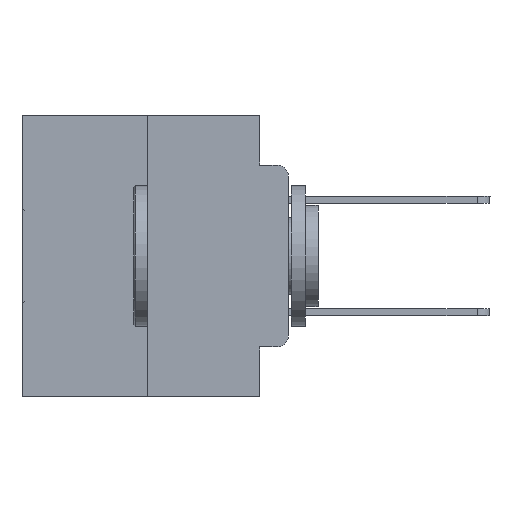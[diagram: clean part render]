
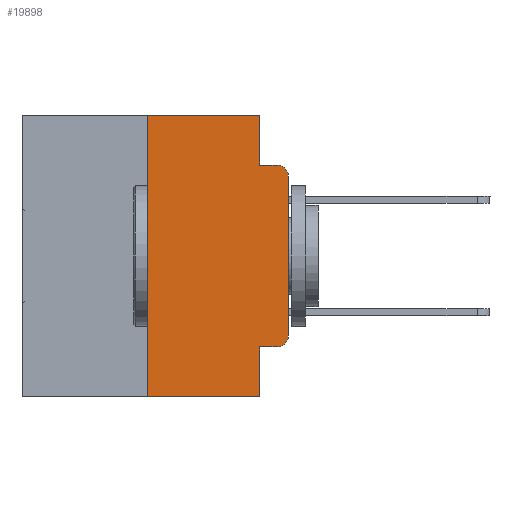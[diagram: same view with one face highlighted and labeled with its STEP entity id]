
A CAD part, left-side view. The second image highlights one B-rep face of the part: STEP entity #19898.
In plain terms, the highlighted planar face has unit normal (-1, 0, 0).
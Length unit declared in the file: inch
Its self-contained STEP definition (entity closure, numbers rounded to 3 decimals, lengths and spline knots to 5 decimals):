
#497 = EDGE_CURVE ( 'NONE', #6407, #11371, #31615, .T. ) ;
#2572 = CARTESIAN_POINT ( 'NONE',  ( 0., 0.02, -0.1085 ) ) ;
#3249 = CARTESIAN_POINT ( 'NONE',  ( 0., 0.473, 0. ) ) ;
#3807 = AXIS2_PLACEMENT_3D ( 'NONE', #2572, #20241, #5185 ) ;
#3982 = CARTESIAN_POINT ( 'NONE',  ( 0., 0.051, 0. ) ) ;
#4073 = CARTESIAN_POINT ( 'NONE',  ( 0., 0.02, -0.0885 ) ) ;
#4460 = VECTOR ( 'NONE', #25792, 39.37008 ) ;
#5185 = DIRECTION ( 'NONE',  ( 0., 0., -1. ) ) ;
#5262 = LINE ( 'NONE', #18296, #4460 ) ;
#5827 = DIRECTION ( 'NONE',  ( 0., 0., -1. ) ) ;
#6192 = VECTOR ( 'NONE', #22529, 39.37008 ) ;
#6322 = VERTEX_POINT ( 'NONE', #23904 ) ;
#6380 = VECTOR ( 'NONE', #16182, 39.37008 ) ;
#6407 = VERTEX_POINT ( 'NONE', #23125 ) ;
#6460 = CARTESIAN_POINT ( 'NONE',  ( 0., 0.25, 0. ) ) ;
#7505 = EDGE_CURVE ( 'NONE', #6407, #19344, #25253, .T. ) ;
#7971 = LINE ( 'NONE', #28502, #6380 ) ;
#8475 = ORIENTED_EDGE ( 'NONE', *, *, #19273, .T. ) ;
#8670 = CARTESIAN_POINT ( 'NONE',  ( 0., 0.051, -0.5 ) ) ;
#8671 = CARTESIAN_POINT ( 'NONE',  ( 0., 0.051, 0. ) ) ;
#8847 = EDGE_CURVE ( 'NONE', #10869, #28067, #17464, .T. ) ;
#9014 = AXIS2_PLACEMENT_3D ( 'NONE', #3249, #20863, #5827 ) ;
#9240 = EDGE_CURVE ( 'NONE', #13804, #10869, #7971, .T. ) ;
#9842 = CARTESIAN_POINT ( 'NONE',  ( 0., 0.473, 0. ) ) ;
#9876 = ORIENTED_EDGE ( 'NONE', *, *, #7505, .F. ) ;
#10343 = DIRECTION ( 'NONE',  ( -1., 0., 0. ) ) ;
#10869 = VERTEX_POINT ( 'NONE', #6460 ) ;
#11147 = CARTESIAN_POINT ( 'NONE',  ( 0., 0.02, -0.4115 ) ) ;
#11371 = VERTEX_POINT ( 'NONE', #11147 ) ;
#11706 = LINE ( 'NONE', #15580, #16750 ) ;
#11901 = VECTOR ( 'NONE', #30129, 39.37008 ) ;
#12413 = DIRECTION ( 'NONE',  ( 0., -1., 0. ) ) ;
#12712 = ORIENTED_EDGE ( 'NONE', *, *, #497, .T. ) ;
#13409 = PLANE ( 'NONE',  #9014 ) ;
#13804 = VERTEX_POINT ( 'NONE', #18641 ) ;
#14194 = VERTEX_POINT ( 'NONE', #17664 ) ;
#14289 = EDGE_CURVE ( 'NONE', #28067, #14194, #11706, .T. ) ;
#15580 = CARTESIAN_POINT ( 'NONE',  ( 0., 0.051, 0. ) ) ;
#15982 = EDGE_CURVE ( 'NONE', #14194, #31257, #5262, .T. ) ;
#16182 = DIRECTION ( 'NONE',  ( 0., 0., 1. ) ) ;
#16750 = VECTOR ( 'NONE', #18080, 39.37008 ) ;
#17464 = LINE ( 'NONE', #9842, #23278 ) ;
#17648 = EDGE_CURVE ( 'NONE', #17913, #31257, #30181, .T. ) ;
#17664 = CARTESIAN_POINT ( 'NONE',  ( 0., 0.051, -0.0885 ) ) ;
#17866 = VECTOR ( 'NONE', #31499, 39.37008 ) ;
#17913 = VERTEX_POINT ( 'NONE', #23844 ) ;
#18080 = DIRECTION ( 'NONE',  ( 0., 0., -1. ) ) ;
#18296 = CARTESIAN_POINT ( 'NONE',  ( 0., 0.051, -0.0885 ) ) ;
#18418 = CARTESIAN_POINT ( 'NONE',  ( 0., 0., 0. ) ) ;
#18641 = CARTESIAN_POINT ( 'NONE',  ( 0., 0.25, -0.5 ) ) ;
#19248 = VECTOR ( 'NONE', #20897, 39.37008 ) ;
#19273 = EDGE_CURVE ( 'NONE', #6322, #17913, #32376, .T. ) ;
#19279 = AXIS2_PLACEMENT_3D ( 'NONE', #25249, #10343, #27712 ) ;
#19344 = VERTEX_POINT ( 'NONE', #8670 ) ;
#19898 = ADVANCED_FACE ( 'NONE', ( #20373 ), #13409, .F. ) ;
#20002 = CARTESIAN_POINT ( 'NONE',  ( 0., 0.473, -0.5 ) ) ;
#20146 = CIRCLE ( 'NONE', #19279, 0.02 ) ;
#20241 = DIRECTION ( 'NONE',  ( -1., 0., 0. ) ) ;
#20329 = LINE ( 'NONE', #20002, #6192 ) ;
#20373 = FACE_OUTER_BOUND ( 'NONE', #24957, .T. ) ;
#20661 = ORIENTED_EDGE ( 'NONE', *, *, #9240, .F. ) ;
#20863 = DIRECTION ( 'NONE',  ( 1., 0., 0. ) ) ;
#20897 = DIRECTION ( 'NONE',  ( 0., 0., 1. ) ) ;
#21380 = EDGE_CURVE ( 'NONE', #13804, #19344, #20329, .T. ) ;
#22116 = ORIENTED_EDGE ( 'NONE', *, *, #14289, .F. ) ;
#22232 = ORIENTED_EDGE ( 'NONE', *, *, #17648, .T. ) ;
#22529 = DIRECTION ( 'NONE',  ( 0., -1., 0. ) ) ;
#23125 = CARTESIAN_POINT ( 'NONE',  ( 0., 0.051, -0.4115 ) ) ;
#23179 = ORIENTED_EDGE ( 'NONE', *, *, #15982, .F. ) ;
#23278 = VECTOR ( 'NONE', #12413, 39.37008 ) ;
#23844 = CARTESIAN_POINT ( 'NONE',  ( 0., 0., -0.1085 ) ) ;
#23904 = CARTESIAN_POINT ( 'NONE',  ( 0., 0., -0.3915 ) ) ;
#24957 = EDGE_LOOP ( 'NONE', ( #8475, #22232, #23179, #22116, #27623, #20661, #26172, #9876, #12712, #31285 ) ) ;
#25249 = CARTESIAN_POINT ( 'NONE',  ( 0., 0.02, -0.3915 ) ) ;
#25253 = LINE ( 'NONE', #3982, #17866 ) ;
#25792 = DIRECTION ( 'NONE',  ( 0., -1., 0. ) ) ;
#26172 = ORIENTED_EDGE ( 'NONE', *, *, #21380, .T. ) ;
#27623 = ORIENTED_EDGE ( 'NONE', *, *, #8847, .F. ) ;
#27712 = DIRECTION ( 'NONE',  ( 0., 0., -1. ) ) ;
#28067 = VERTEX_POINT ( 'NONE', #8671 ) ;
#28502 = CARTESIAN_POINT ( 'NONE',  ( 0., 0.25, 0. ) ) ;
#30129 = DIRECTION ( 'NONE',  ( 0., -1., 0. ) ) ;
#30181 = CIRCLE ( 'NONE', #3807, 0.02 ) ;
#31257 = VERTEX_POINT ( 'NONE', #4073 ) ;
#31285 = ORIENTED_EDGE ( 'NONE', *, *, #31495, .T. ) ;
#31495 = EDGE_CURVE ( 'NONE', #11371, #6322, #20146, .T. ) ;
#31499 = DIRECTION ( 'NONE',  ( 0., 0., -1. ) ) ;
#31615 = LINE ( 'NONE', #32117, #11901 ) ;
#32117 = CARTESIAN_POINT ( 'NONE',  ( 0., 0.051, -0.4115 ) ) ;
#32376 = LINE ( 'NONE', #18418, #19248 ) ;
